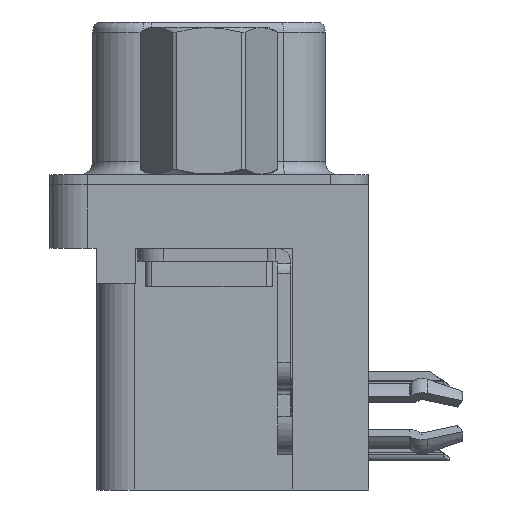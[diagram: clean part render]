
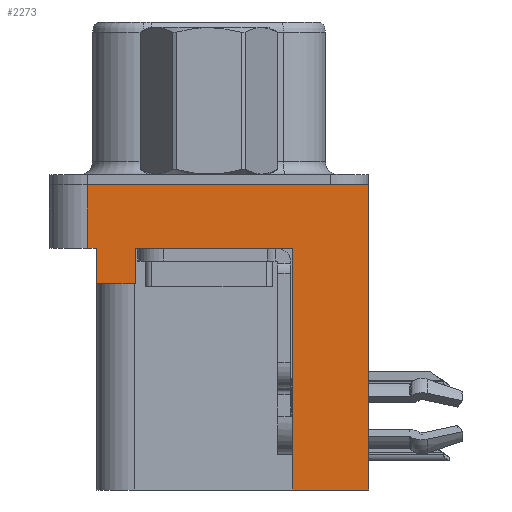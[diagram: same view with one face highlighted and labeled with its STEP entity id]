
A CAD part, left-side view. The second image highlights one B-rep face of the part: STEP entity #2273.
In plain terms, the highlighted planar face has unit normal (-1, 0, 0).
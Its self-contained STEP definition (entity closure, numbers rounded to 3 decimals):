
#100 = DIRECTION ( 'NONE',  ( 0., 1., 0. ) ) ;
#482 = EDGE_CURVE ( 'NONE', #4010, #8977, #13441, .T. ) ;
#681 = LINE ( 'NONE', #3875, #29526 ) ;
#817 = CARTESIAN_POINT ( 'NONE',  ( -3., -6.275, -2.5 ) ) ;
#1503 = VECTOR ( 'NONE', #9589, 1000. ) ;
#1511 = VERTEX_POINT ( 'NONE', #23094 ) ;
#1894 = EDGE_CURVE ( 'NONE', #23463, #22613, #22605, .T. ) ;
#2088 = CARTESIAN_POINT ( 'NONE',  ( -3., -3.295, -12. ) ) ;
#2155 = CARTESIAN_POINT ( 'NONE',  ( -3., -6.275, 0. ) ) ;
#2273 = ADVANCED_FACE ( 'NONE', ( #17936 ), #8900, .T. ) ;
#2662 = LINE ( 'NONE', #2088, #4469 ) ;
#3081 = VERTEX_POINT ( 'NONE', #28359 ) ;
#3274 = ORIENTED_EDGE ( 'NONE', *, *, #14750, .F. ) ;
#3875 = CARTESIAN_POINT ( 'NONE',  ( -3., -6.275, -2.5 ) ) ;
#4010 = VERTEX_POINT ( 'NONE', #7816 ) ;
#4203 = CARTESIAN_POINT ( 'NONE',  ( -3., 4.425, -2.5 ) ) ;
#4205 = VECTOR ( 'NONE', #20478, 1000. ) ;
#4278 = LINE ( 'NONE', #817, #9568 ) ;
#4469 = VECTOR ( 'NONE', #8764, 1000. ) ;
#4576 = CARTESIAN_POINT ( 'NONE',  ( -3., 2.895, -2.5 ) ) ;
#4685 = DIRECTION ( 'NONE',  ( 0., 1., 0. ) ) ;
#5129 = DIRECTION ( 'NONE',  ( 0., -1., 0. ) ) ;
#5197 = VERTEX_POINT ( 'NONE', #4576 ) ;
#6837 = DIRECTION ( 'NONE',  ( 0., 0., 1. ) ) ;
#7056 = EDGE_LOOP ( 'NONE', ( #25728, #24653, #22934, #11918, #3274, #9857, #22482, #15444, #8579, #15303 ) ) ;
#7506 = EDGE_CURVE ( 'NONE', #27784, #1511, #9291, .T. ) ;
#7816 = CARTESIAN_POINT ( 'NONE',  ( -3., 4.775, -2.5 ) ) ;
#8285 = EDGE_CURVE ( 'NONE', #5197, #20687, #4278, .T. ) ;
#8579 = ORIENTED_EDGE ( 'NONE', *, *, #7506, .F. ) ;
#8764 = DIRECTION ( 'NONE',  ( 0., 0., 1. ) ) ;
#8776 = CARTESIAN_POINT ( 'NONE',  ( -3., -6.275, 0. ) ) ;
#8870 = DIRECTION ( 'NONE',  ( 0., -1., 0. ) ) ;
#8900 = PLANE ( 'NONE',  #20587 ) ;
#8977 = VERTEX_POINT ( 'NONE', #4203 ) ;
#9291 = LINE ( 'NONE', #27148, #11112 ) ;
#9568 = VECTOR ( 'NONE', #5129, 1000. ) ;
#9589 = DIRECTION ( 'NONE',  ( 0., 0., 1. ) ) ;
#9857 = ORIENTED_EDGE ( 'NONE', *, *, #18526, .T. ) ;
#10469 = VECTOR ( 'NONE', #18730, 1000. ) ;
#11112 = VECTOR ( 'NONE', #100, 1000. ) ;
#11335 = EDGE_CURVE ( 'NONE', #1511, #20687, #2662, .T. ) ;
#11918 = ORIENTED_EDGE ( 'NONE', *, *, #14669, .F. ) ;
#13441 = LINE ( 'NONE', #27245, #4205 ) ;
#14535 = VECTOR ( 'NONE', #17581, 1000. ) ;
#14669 = EDGE_CURVE ( 'NONE', #3081, #8977, #22715, .T. ) ;
#14750 = EDGE_CURVE ( 'NONE', #15935, #3081, #18620, .T. ) ;
#15303 = ORIENTED_EDGE ( 'NONE', *, *, #23886, .T. ) ;
#15444 = ORIENTED_EDGE ( 'NONE', *, *, #11335, .F. ) ;
#15787 = LINE ( 'NONE', #20442, #10469 ) ;
#15935 = VERTEX_POINT ( 'NONE', #18790 ) ;
#16851 = CARTESIAN_POINT ( 'NONE',  ( -3., -3.295, -2.5 ) ) ;
#17256 = VECTOR ( 'NONE', #8870, 1000. ) ;
#17581 = DIRECTION ( 'NONE',  ( 0., 0., 1. ) ) ;
#17936 = FACE_OUTER_BOUND ( 'NONE', #7056, .T. ) ;
#18270 = CARTESIAN_POINT ( 'NONE',  ( -3., 4.425, -3.9 ) ) ;
#18526 = EDGE_CURVE ( 'NONE', #15935, #5197, #15787, .T. ) ;
#18620 = LINE ( 'NONE', #18270, #22236 ) ;
#18730 = DIRECTION ( 'NONE',  ( 0., 0., 1. ) ) ;
#18790 = CARTESIAN_POINT ( 'NONE',  ( -3., 2.895, -3.9 ) ) ;
#19502 = CARTESIAN_POINT ( 'NONE',  ( -3., -6.275, -12. ) ) ;
#20389 = CARTESIAN_POINT ( 'NONE',  ( -3., -6.275, -2.5 ) ) ;
#20442 = CARTESIAN_POINT ( 'NONE',  ( -3., 2.895, -3.9 ) ) ;
#20478 = DIRECTION ( 'NONE',  ( 0., -1., 0. ) ) ;
#20587 = AXIS2_PLACEMENT_3D ( 'NONE', #20389, #26762, #6837 ) ;
#20687 = VERTEX_POINT ( 'NONE', #16851 ) ;
#20916 = CARTESIAN_POINT ( 'NONE',  ( -3., 4.775, -2.5 ) ) ;
#22236 = VECTOR ( 'NONE', #4685, 1000. ) ;
#22482 = ORIENTED_EDGE ( 'NONE', *, *, #8285, .T. ) ;
#22605 = LINE ( 'NONE', #8776, #17256 ) ;
#22613 = VERTEX_POINT ( 'NONE', #2155 ) ;
#22715 = LINE ( 'NONE', #28964, #14535 ) ;
#22934 = ORIENTED_EDGE ( 'NONE', *, *, #482, .T. ) ;
#23094 = CARTESIAN_POINT ( 'NONE',  ( -3., -3.295, -12. ) ) ;
#23463 = VERTEX_POINT ( 'NONE', #24357 ) ;
#23886 = EDGE_CURVE ( 'NONE', #27784, #22613, #681, .T. ) ;
#24357 = CARTESIAN_POINT ( 'NONE',  ( -3., 4.775, 0. ) ) ;
#24653 = ORIENTED_EDGE ( 'NONE', *, *, #27632, .F. ) ;
#25728 = ORIENTED_EDGE ( 'NONE', *, *, #1894, .F. ) ;
#26762 = DIRECTION ( 'NONE',  ( -1., 0., 0. ) ) ;
#27148 = CARTESIAN_POINT ( 'NONE',  ( -3., -3.295, -12. ) ) ;
#27245 = CARTESIAN_POINT ( 'NONE',  ( -3., -6.275, -2.5 ) ) ;
#27632 = EDGE_CURVE ( 'NONE', #4010, #23463, #27806, .T. ) ;
#27784 = VERTEX_POINT ( 'NONE', #19502 ) ;
#27806 = LINE ( 'NONE', #20916, #1503 ) ;
#28359 = CARTESIAN_POINT ( 'NONE',  ( -3., 4.425, -3.9 ) ) ;
#28943 = DIRECTION ( 'NONE',  ( 0., 0., 1. ) ) ;
#28964 = CARTESIAN_POINT ( 'NONE',  ( -3., 4.425, -3.9 ) ) ;
#29526 = VECTOR ( 'NONE', #28943, 1000. ) ;
